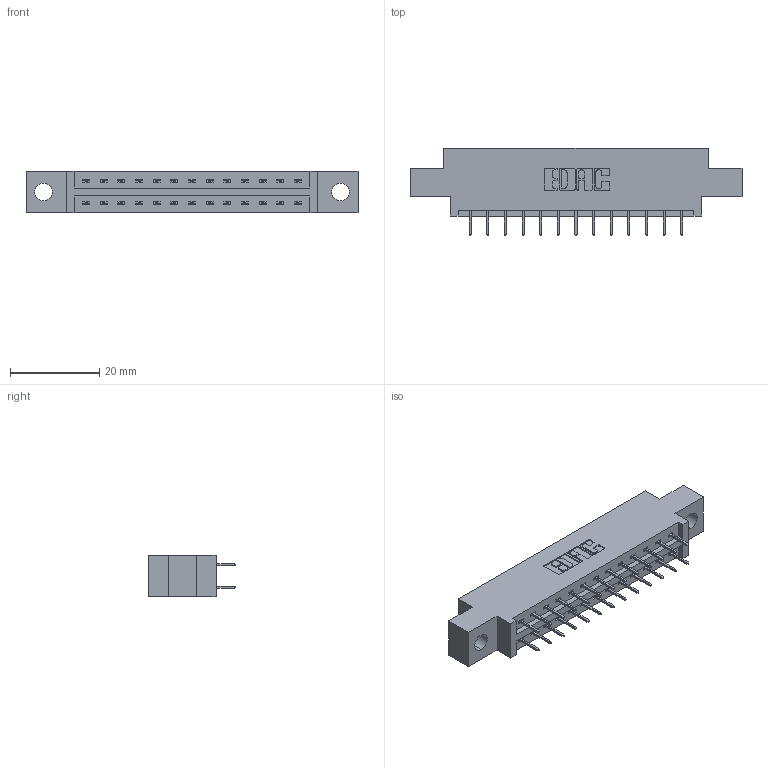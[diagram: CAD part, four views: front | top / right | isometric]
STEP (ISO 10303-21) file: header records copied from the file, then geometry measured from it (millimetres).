
FILE_DESCRIPTION (( 'STEP AP203' ), '1' );
FILE_NAME ('387-026-524-804.STEP', '2019-10-16T19:52:12', ( '' ), ( '' ), 'SwSTEP 2.0', 'SolidWorks 2016', '' );
FILE_SCHEMA (( 'CONFIG_CONTROL_DESIGN' ));
Length unit declared in the file: inch
Products named in the file (3): 337 Part_0.170 Offset - 0.156 Dia-TH; 345-292-001_345-293-124; 387-026-524-804
Assembly tree (27 placements, depth 2):
  387-026-524-804
    337 Part_0.170 Offset - 0.156 Dia-TH
    345-292-001_345-293-124  x26
Bounding box: 74.52 x 19.69 x 9.4 mm (x, y, z)
Volume: 7223.2 mm3; surface area: 7667.5 mm2
Topology: 27 solids, 27 shells, 1626 faces, 4613 edges, 2970 vertices
Faces by surface type: plane 1218, cylinder 408
Entity records: 14039 total; most frequent: CARTESIAN_POINT 2390, ORIENTED_EDGE 2326, DIRECTION 2087, EDGE_CURVE 1163, VECTOR 1039, LINE 1039, VERTEX_POINT 770, AXIS2_PLACEMENT_3D 524
